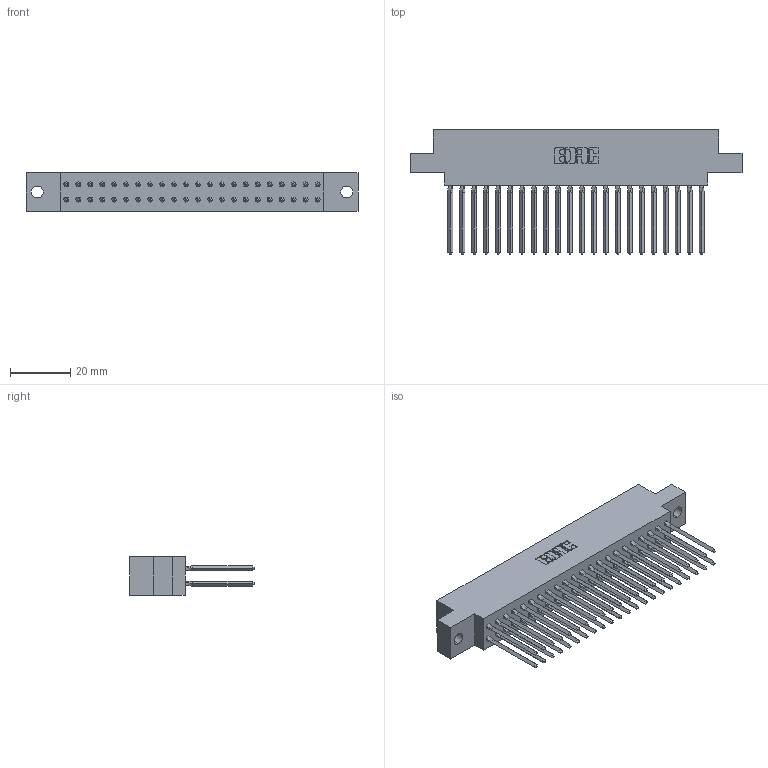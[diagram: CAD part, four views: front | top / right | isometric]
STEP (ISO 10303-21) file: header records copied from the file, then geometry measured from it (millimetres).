
FILE_DESCRIPTION (( 'STEP AP203' ), '1' );
FILE_NAME ('317-044-543-804.STEP', '2020-02-28T02:13:43', ( '' ), ( '' ), 'SwSTEP 2.0', 'SolidWorks 2016', '' );
FILE_SCHEMA (( 'CONFIG_CONTROL_DESIGN' ));
Length unit declared in the file: inch
Products named in the file (3): 317-290-001_543; 317-044-543-804; 317 Part_.156 Dia - TH
Assembly tree (45 placements, depth 2):
  317-044-543-804
    317 Part_.156 Dia - TH
    317-290-001_543  x44
Bounding box: 109.88 x 41.15 x 12.7 mm (x, y, z)
Volume: 17896.3 mm3; surface area: 26191.2 mm2
Topology: 45 solids, 45 shells, 4018 faces, 11143 edges, 7178 vertices
Faces by surface type: plane 3270, cylinder 572, bspline 176
Entity records: 34594 total; most frequent: CARTESIAN_POINT 6447, ORIENTED_EDGE 5946, DIRECTION 4963, EDGE_CURVE 2973, VECTOR 2717, LINE 2717, VERTEX_POINT 1975, AXIS2_PLACEMENT_3D 1123
